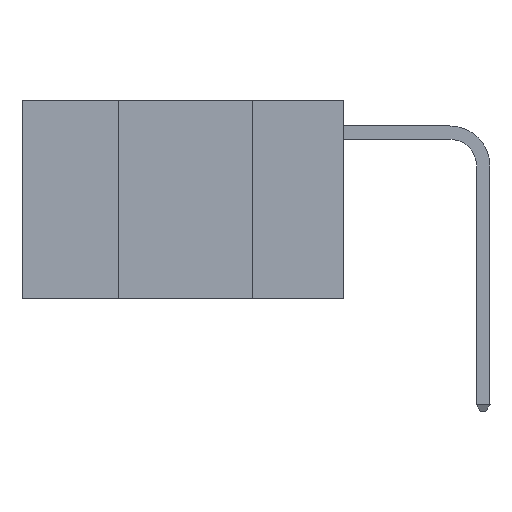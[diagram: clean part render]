
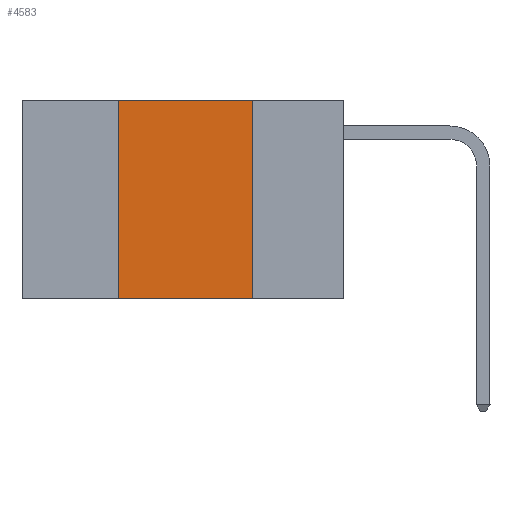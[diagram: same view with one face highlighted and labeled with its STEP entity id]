
A CAD part, left-side view. The second image highlights one B-rep face of the part: STEP entity #4583.
In plain terms, the highlighted planar face has unit normal (-1, 0, 0).
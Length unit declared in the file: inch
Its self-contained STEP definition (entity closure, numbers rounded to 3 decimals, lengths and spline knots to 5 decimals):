
#32 = CARTESIAN_POINT ( 'NONE',  ( 0., 0.6, 0. ) ) ;
#744 = DIRECTION ( 'NONE',  ( 0., 0., 1. ) ) ;
#966 = CARTESIAN_POINT ( 'NONE',  ( 0., 0.17, 0. ) ) ;
#1049 = VECTOR ( 'NONE', #744, 39.37008 ) ;
#1596 = DIRECTION ( 'NONE',  ( 0., 0., -1. ) ) ;
#1598 = FACE_OUTER_BOUND ( 'NONE', #3986, .T. ) ;
#3747 = VECTOR ( 'NONE', #1596, 39.37008 ) ;
#3986 = EDGE_LOOP ( 'NONE', ( #4345, #24888, #11203, #27982 ) ) ;
#4345 = ORIENTED_EDGE ( 'NONE', *, *, #11315, .F. ) ;
#4500 = DIRECTION ( 'NONE',  ( 1., 0., 0. ) ) ;
#4583 = ADVANCED_FACE ( 'NONE', ( #1598 ), #17609, .F. ) ;
#4665 = DIRECTION ( 'NONE',  ( 0., -1., 0. ) ) ;
#6843 = VECTOR ( 'NONE', #4665, 39.37008 ) ;
#10462 = CARTESIAN_POINT ( 'NONE',  ( 0., 0.42, -0.37 ) ) ;
#11203 = ORIENTED_EDGE ( 'NONE', *, *, #21374, .F. ) ;
#11226 = LINE ( 'NONE', #23108, #16351 ) ;
#11315 = EDGE_CURVE ( 'NONE', #19461, #17489, #17464, .T. ) ;
#12543 = VERTEX_POINT ( 'NONE', #10462 ) ;
#12663 = LINE ( 'NONE', #19977, #6843 ) ;
#13462 = LINE ( 'NONE', #20527, #1049 ) ;
#16351 = VECTOR ( 'NONE', #23197, 39.37008 ) ;
#16972 = CARTESIAN_POINT ( 'NONE',  ( 0., 0.17, 0. ) ) ;
#17062 = EDGE_CURVE ( 'NONE', #17219, #19461, #12663, .T. ) ;
#17219 = VERTEX_POINT ( 'NONE', #20348 ) ;
#17464 = LINE ( 'NONE', #16972, #3747 ) ;
#17489 = VERTEX_POINT ( 'NONE', #25167 ) ;
#17609 = PLANE ( 'NONE',  #27978 ) ;
#18230 = EDGE_CURVE ( 'NONE', #12543, #17489, #11226, .T. ) ;
#19461 = VERTEX_POINT ( 'NONE', #966 ) ;
#19805 = DIRECTION ( 'NONE',  ( 0., 0., -1. ) ) ;
#19977 = CARTESIAN_POINT ( 'NONE',  ( 0., 0.6, 0. ) ) ;
#20348 = CARTESIAN_POINT ( 'NONE',  ( 0., 0.42, 0. ) ) ;
#20527 = CARTESIAN_POINT ( 'NONE',  ( 0., 0.42, 0. ) ) ;
#21374 = EDGE_CURVE ( 'NONE', #12543, #17219, #13462, .T. ) ;
#23108 = CARTESIAN_POINT ( 'NONE',  ( 0., 0.6, -0.37 ) ) ;
#23197 = DIRECTION ( 'NONE',  ( 0., -1., 0. ) ) ;
#24888 = ORIENTED_EDGE ( 'NONE', *, *, #17062, .F. ) ;
#25167 = CARTESIAN_POINT ( 'NONE',  ( 0., 0.17, -0.37 ) ) ;
#27978 = AXIS2_PLACEMENT_3D ( 'NONE', #32, #4500, #19805 ) ;
#27982 = ORIENTED_EDGE ( 'NONE', *, *, #18230, .T. ) ;
